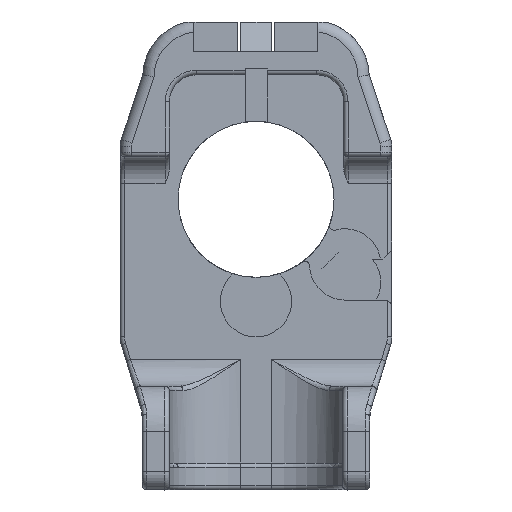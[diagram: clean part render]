
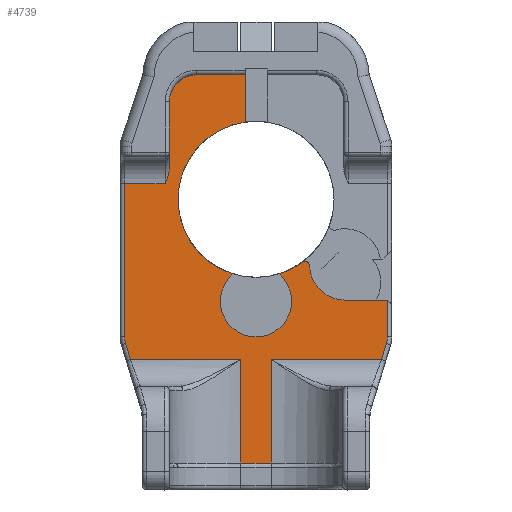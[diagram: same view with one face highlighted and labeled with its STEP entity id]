
A CAD part, front view. The second image highlights one B-rep face of the part: STEP entity #4739.
In plain terms, the highlighted planar face has unit normal (0, -1, 0).
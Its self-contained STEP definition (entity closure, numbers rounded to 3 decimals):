
#263=B_SPLINE_CURVE_WITH_KNOTS('',3,(#8817,#8818,#8819,#8820),
 .UNSPECIFIED.,.F.,.F.,(4,4),(0.382,0.56),
 .UNSPECIFIED.);
#400=PLANE('',#5077);
#563=FACE_OUTER_BOUND('',#851,.T.);
#851=EDGE_LOOP('',(#3836,#3837,#3838,#3839,#3840,#3841,#3842,#3843,#3844,
#3845,#3846,#3847,#3848,#3849,#3850,#3851,#3852,#3853,#3854,#3855,#3856,
#3857,#3858));
#1053=CIRCLE('',#5043,8.75);
#1055=CIRCLE('',#5045,8.75);
#1064=CIRCLE('',#5075,3.);
#1066=CIRCLE('',#5078,2.5);
#1067=CIRCLE('',#5079,2.5);
#1068=CIRCLE('',#5080,4.);
#1069=CIRCLE('',#5081,0.5);
#1070=CIRCLE('',#5082,4.);
#1442=LINE('',#8790,#1832);
#1444=LINE('',#8794,#1834);
#1450=LINE('',#8815,#1840);
#1451=LINE('',#8822,#1841);
#1452=LINE('',#8824,#1842);
#1453=LINE('',#8828,#1843);
#1454=LINE('',#8830,#1844);
#1455=LINE('',#8832,#1845);
#1456=LINE('',#8834,#1846);
#1457=LINE('',#8836,#1847);
#1458=LINE('',#8838,#1848);
#1459=LINE('',#8840,#1849);
#1460=LINE('',#8844,#1850);
#1461=LINE('',#8846,#1851);
#1832=VECTOR('',#5913,10.);
#1834=VECTOR('',#5917,10.);
#1840=VECTOR('',#5937,10.);
#1841=VECTOR('',#5938,10.);
#1842=VECTOR('',#5939,10.);
#1843=VECTOR('',#5942,10.);
#1844=VECTOR('',#5943,10.);
#1845=VECTOR('',#5944,10.);
#1846=VECTOR('',#5945,10.);
#1847=VECTOR('',#5946,10.);
#1848=VECTOR('',#5947,10.);
#1849=VECTOR('',#5948,10.);
#1850=VECTOR('',#5951,10.);
#1851=VECTOR('',#5952,10.);
#2242=VERTEX_POINT('',#8624);
#2243=VERTEX_POINT('',#8626);
#2246=VERTEX_POINT('',#8632);
#2247=VERTEX_POINT('',#8634);
#2263=VERTEX_POINT('',#8788);
#2264=VERTEX_POINT('',#8793);
#2270=VERTEX_POINT('',#8808);
#2272=VERTEX_POINT('',#8814);
#2273=VERTEX_POINT('',#8816);
#2274=VERTEX_POINT('',#8821);
#2275=VERTEX_POINT('',#8823);
#2276=VERTEX_POINT('',#8825);
#2277=VERTEX_POINT('',#8827);
#2278=VERTEX_POINT('',#8829);
#2279=VERTEX_POINT('',#8831);
#2280=VERTEX_POINT('',#8833);
#2281=VERTEX_POINT('',#8835);
#2282=VERTEX_POINT('',#8837);
#2283=VERTEX_POINT('',#8839);
#2284=VERTEX_POINT('',#8841);
#2285=VERTEX_POINT('',#8843);
#2286=VERTEX_POINT('',#8845);
#2287=VERTEX_POINT('',#8847);
#2786=EDGE_CURVE('',#2243,#2242,#1053,.T.);
#2790=EDGE_CURVE('',#2247,#2246,#1055,.T.);
#2824=EDGE_CURVE('',#2263,#2242,#1442,.T.);
#2826=EDGE_CURVE('',#2263,#2264,#1444,.T.);
#2833=EDGE_CURVE('',#2264,#2270,#1064,.T.);
#2836=EDGE_CURVE('',#2270,#2272,#1450,.T.);
#2837=EDGE_CURVE('',#2273,#2272,#263,.F.);
#2838=EDGE_CURVE('',#2274,#2273,#1451,.T.);
#2839=EDGE_CURVE('',#2275,#2274,#1452,.T.);
#2840=EDGE_CURVE('',#2276,#2275,#1066,.T.);
#2841=EDGE_CURVE('',#2277,#2276,#1453,.T.);
#2842=EDGE_CURVE('',#2277,#2278,#1454,.T.);
#2843=EDGE_CURVE('',#2279,#2278,#1455,.T.);
#2844=EDGE_CURVE('',#2279,#2280,#1456,.T.);
#2845=EDGE_CURVE('',#2281,#2280,#1457,.T.);
#2846=EDGE_CURVE('',#2281,#2282,#1458,.T.);
#2847=EDGE_CURVE('',#2283,#2282,#1459,.T.);
#2848=EDGE_CURVE('',#2284,#2283,#1067,.T.);
#2849=EDGE_CURVE('',#2285,#2284,#1460,.T.);
#2850=EDGE_CURVE('',#2286,#2285,#1461,.T.);
#2851=EDGE_CURVE('',#2286,#2287,#1068,.T.);
#2852=EDGE_CURVE('',#2247,#2287,#1069,.T.);
#2853=EDGE_CURVE('',#2246,#2243,#1070,.T.);
#3836=ORIENTED_EDGE('',*,*,#2833,.T.);
#3837=ORIENTED_EDGE('',*,*,#2836,.T.);
#3838=ORIENTED_EDGE('',*,*,#2837,.F.);
#3839=ORIENTED_EDGE('',*,*,#2838,.F.);
#3840=ORIENTED_EDGE('',*,*,#2839,.F.);
#3841=ORIENTED_EDGE('',*,*,#2840,.F.);
#3842=ORIENTED_EDGE('',*,*,#2841,.F.);
#3843=ORIENTED_EDGE('',*,*,#2842,.T.);
#3844=ORIENTED_EDGE('',*,*,#2843,.F.);
#3845=ORIENTED_EDGE('',*,*,#2844,.T.);
#3846=ORIENTED_EDGE('',*,*,#2845,.F.);
#3847=ORIENTED_EDGE('',*,*,#2846,.T.);
#3848=ORIENTED_EDGE('',*,*,#2847,.F.);
#3849=ORIENTED_EDGE('',*,*,#2848,.F.);
#3850=ORIENTED_EDGE('',*,*,#2849,.F.);
#3851=ORIENTED_EDGE('',*,*,#2850,.F.);
#3852=ORIENTED_EDGE('',*,*,#2851,.T.);
#3853=ORIENTED_EDGE('',*,*,#2852,.F.);
#3854=ORIENTED_EDGE('',*,*,#2790,.T.);
#3855=ORIENTED_EDGE('',*,*,#2853,.T.);
#3856=ORIENTED_EDGE('',*,*,#2786,.T.);
#3857=ORIENTED_EDGE('',*,*,#2824,.F.);
#3858=ORIENTED_EDGE('',*,*,#2826,.T.);
#4739=ADVANCED_FACE('',(#563),#400,.T.);
#5043=AXIS2_PLACEMENT_3D('',#8627,#5835,#5836);
#5045=AXIS2_PLACEMENT_3D('',#8635,#5841,#5842);
#5075=AXIS2_PLACEMENT_3D('',#8809,#5930,#5931);
#5077=AXIS2_PLACEMENT_3D('',#8813,#5935,#5936);
#5078=AXIS2_PLACEMENT_3D('',#8826,#5940,#5941);
#5079=AXIS2_PLACEMENT_3D('',#8842,#5949,#5950);
#5080=AXIS2_PLACEMENT_3D('',#8848,#5953,#5954);
#5081=AXIS2_PLACEMENT_3D('',#8849,#5955,#5956);
#5082=AXIS2_PLACEMENT_3D('',#8850,#5957,#5958);
#5835=DIRECTION('center_axis',(0.,1.,0.));
#5836=DIRECTION('ref_axis',(-1.,0.,0.));
#5841=DIRECTION('center_axis',(0.,1.,0.));
#5842=DIRECTION('ref_axis',(-1.,0.,0.));
#5913=DIRECTION('',(0.,0.,-1.));
#5917=DIRECTION('',(-1.,0.,0.));
#5930=DIRECTION('center_axis',(0.,-1.,0.));
#5931=DIRECTION('ref_axis',(-1.,0.,0.));
#5935=DIRECTION('center_axis',(0.,-1.,0.));
#5936=DIRECTION('ref_axis',(0.,0.,-1.));
#5937=DIRECTION('',(0.,0.,-1.));
#5938=DIRECTION('',(1.,0.,0.));
#5939=DIRECTION('',(0.,0.,1.));
#5940=DIRECTION('center_axis',(0.,1.,0.));
#5941=DIRECTION('ref_axis',(-0.989,0.,-0.149));
#5942=DIRECTION('',(-0.294,0.,0.956));
#5943=DIRECTION('',(1.,0.,0.));
#5944=DIRECTION('',(0.,0.,1.));
#5945=DIRECTION('',(1.,0.,0.));
#5946=DIRECTION('',(0.,0.,-1.));
#5947=DIRECTION('',(1.,0.,0.));
#5948=DIRECTION('',(-0.294,0.,-0.956));
#5949=DIRECTION('center_axis',(0.,1.,0.));
#5950=DIRECTION('ref_axis',(0.989,0.,-0.149));
#5951=DIRECTION('',(0.,0.,-1.));
#5952=DIRECTION('',(1.,0.,0.));
#5953=DIRECTION('center_axis',(0.,1.,0.));
#5954=DIRECTION('ref_axis',(-0.751,0.,0.66));
#5955=DIRECTION('center_axis',(0.,1.,0.));
#5956=DIRECTION('ref_axis',(0.437,0.,0.9));
#5957=DIRECTION('center_axis',(0.,1.,0.));
#5958=DIRECTION('ref_axis',(1.,0.,0.));
#8624=CARTESIAN_POINT('',(-1.212,65.024,-354.904));
#8626=CARTESIAN_POINT('',(-2.569,65.024,-371.934));
#8627=CARTESIAN_POINT('Origin',(0.,65.024,-363.57));
#8632=CARTESIAN_POINT('',(2.569,65.024,-371.934));
#8634=CARTESIAN_POINT('',(5.205,65.024,-370.604));
#8635=CARTESIAN_POINT('Origin',(0.,65.024,-363.57));
#8788=CARTESIAN_POINT('',(-1.212,65.024,-349.606));
#8790=CARTESIAN_POINT('',(-1.212,65.024,-361.281));
#8793=CARTESIAN_POINT('',(-6.692,65.024,-349.606));
#8794=CARTESIAN_POINT('',(-12.701,65.024,-349.606));
#8808=CARTESIAN_POINT('',(-9.692,65.024,-352.606));
#8809=CARTESIAN_POINT('Origin',(-6.692,65.024,-352.606));
#8813=CARTESIAN_POINT('Origin',(-12.7,65.024,-367.382));
#8814=CARTESIAN_POINT('',(-9.692,65.024,-360.002));
#8815=CARTESIAN_POINT('',(-9.692,65.024,-363.093));
#8816=CARTESIAN_POINT('',(-10.192,65.024,-361.805));
#8817=CARTESIAN_POINT('Ctrl Pts',(-9.692,65.024,-360.002));
#8818=CARTESIAN_POINT('Ctrl Pts',(-9.692,65.024,-360.597));
#8819=CARTESIAN_POINT('Ctrl Pts',(-9.968,65.024,-361.255));
#8820=CARTESIAN_POINT('Ctrl Pts',(-10.192,65.024,-361.805));
#8821=CARTESIAN_POINT('',(-14.74,65.024,-361.805));
#8822=CARTESIAN_POINT('',(-13.97,65.024,-361.805));
#8823=CARTESIAN_POINT('',(-14.74,65.024,-378.994));
#8824=CARTESIAN_POINT('',(-14.74,65.024,-365.95));
#8825=CARTESIAN_POINT('',(-14.629,65.024,-379.729));
#8826=CARTESIAN_POINT('Origin',(-12.24,65.024,-378.994));
#8827=CARTESIAN_POINT('',(-14.077,65.024,-381.525));
#8828=CARTESIAN_POINT('',(-15.078,65.024,-378.272));
#8829=CARTESIAN_POINT('',(-1.723,65.024,-381.525));
#8830=CARTESIAN_POINT('',(-10.795,65.024,-381.525));
#8831=CARTESIAN_POINT('',(-1.723,65.024,-393.145));
#8832=CARTESIAN_POINT('',(-1.723,65.024,-383.763));
#8833=CARTESIAN_POINT('',(1.723,65.024,-393.145));
#8834=CARTESIAN_POINT('',(-6.35,65.024,-393.145));
#8835=CARTESIAN_POINT('',(1.723,65.024,-381.525));
#8836=CARTESIAN_POINT('',(1.723,65.024,-376.066));
#8837=CARTESIAN_POINT('',(14.077,65.024,-381.525));
#8838=CARTESIAN_POINT('',(1.27,65.024,-381.525));
#8839=CARTESIAN_POINT('',(14.629,65.024,-379.729));
#8840=CARTESIAN_POINT('',(16.519,65.024,-373.587));
#8841=CARTESIAN_POINT('',(14.74,65.024,-378.994));
#8842=CARTESIAN_POINT('Origin',(12.24,65.024,-378.994));
#8843=CARTESIAN_POINT('',(14.74,65.024,-374.871));
#8844=CARTESIAN_POINT('',(14.74,65.024,-365.945));
#8845=CARTESIAN_POINT('',(9.906,65.024,-374.871));
#8846=CARTESIAN_POINT('',(9.953,65.024,-374.871));
#8847=CARTESIAN_POINT('',(6.002,65.024,-370.991));
#8848=CARTESIAN_POINT('Origin',(10.,65.024,-370.872));
#8849=CARTESIAN_POINT('Origin',(5.502,65.024,-371.006));
#8850=CARTESIAN_POINT('Origin',(0.,65.024,-375.));
